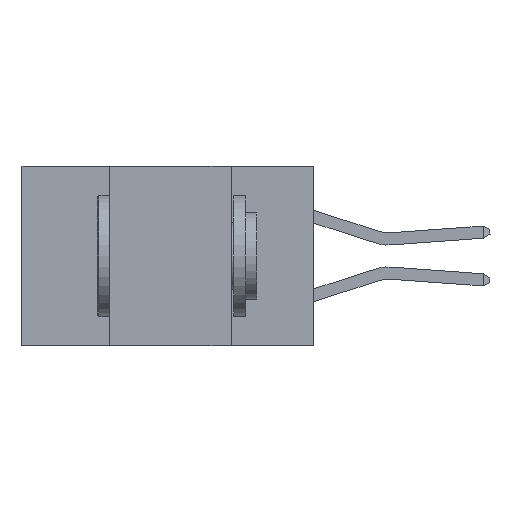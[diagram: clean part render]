
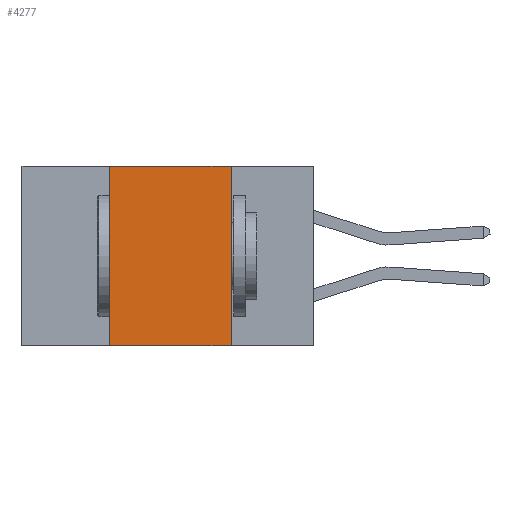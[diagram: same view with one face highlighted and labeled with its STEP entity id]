
A CAD part, left-side view. The second image highlights one B-rep face of the part: STEP entity #4277.
In plain terms, the highlighted planar face has unit normal (-1, 0, 0).
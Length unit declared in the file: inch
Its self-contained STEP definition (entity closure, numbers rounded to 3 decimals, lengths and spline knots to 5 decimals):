
#443 = EDGE_CURVE ( 'NONE', #3996, #13075, #4246, .T. ) ;
#648 = AXIS2_PLACEMENT_3D ( 'NONE', #6887, #17113, #2607 ) ;
#1270 = CARTESIAN_POINT ( 'NONE',  ( 0., 0.17, 0. ) ) ;
#2012 = CARTESIAN_POINT ( 'NONE',  ( 0., 0.6, 0. ) ) ;
#2023 = EDGE_LOOP ( 'NONE', ( #3875, #4181, #4690, #10925 ) ) ;
#2097 = EDGE_CURVE ( 'NONE', #2943, #5993, #6501, .T. ) ;
#2547 = PLANE ( 'NONE',  #648 ) ;
#2607 = DIRECTION ( 'NONE',  ( 0., 0., -1. ) ) ;
#2943 = VERTEX_POINT ( 'NONE', #13710 ) ;
#3200 = CARTESIAN_POINT ( 'NONE',  ( 0., 0.17, 0. ) ) ;
#3426 = DIRECTION ( 'NONE',  ( 0., -1., 0. ) ) ;
#3869 = DIRECTION ( 'NONE',  ( 0., 0., 1. ) ) ;
#3875 = ORIENTED_EDGE ( 'NONE', *, *, #443, .F. ) ;
#3996 = VERTEX_POINT ( 'NONE', #3200 ) ;
#4126 = VECTOR ( 'NONE', #3426, 39.37008 ) ;
#4181 = ORIENTED_EDGE ( 'NONE', *, *, #14505, .F. ) ;
#4246 = LINE ( 'NONE', #1270, #5162 ) ;
#4277 = ADVANCED_FACE ( 'NONE', ( #12314 ), #2547, .F. ) ;
#4450 = CARTESIAN_POINT ( 'NONE',  ( 0., 0.42, 0. ) ) ;
#4690 = ORIENTED_EDGE ( 'NONE', *, *, #2097, .F. ) ;
#5162 = VECTOR ( 'NONE', #14356, 39.37008 ) ;
#5337 = VECTOR ( 'NONE', #7429, 39.37008 ) ;
#5881 = CARTESIAN_POINT ( 'NONE',  ( 0., 0.17, -0.37 ) ) ;
#5993 = VERTEX_POINT ( 'NONE', #4450 ) ;
#6501 = LINE ( 'NONE', #15559, #14306 ) ;
#6887 = CARTESIAN_POINT ( 'NONE',  ( 0., 0.6, 0. ) ) ;
#7429 = DIRECTION ( 'NONE',  ( 0., -1., 0. ) ) ;
#8698 = CARTESIAN_POINT ( 'NONE',  ( 0., 0.6, -0.37 ) ) ;
#10925 = ORIENTED_EDGE ( 'NONE', *, *, #17658, .T. ) ;
#12314 = FACE_OUTER_BOUND ( 'NONE', #2023, .T. ) ;
#13075 = VERTEX_POINT ( 'NONE', #5881 ) ;
#13710 = CARTESIAN_POINT ( 'NONE',  ( 0., 0.42, -0.37 ) ) ;
#14306 = VECTOR ( 'NONE', #3869, 39.37008 ) ;
#14356 = DIRECTION ( 'NONE',  ( 0., 0., -1. ) ) ;
#14505 = EDGE_CURVE ( 'NONE', #5993, #3996, #18591, .T. ) ;
#15559 = CARTESIAN_POINT ( 'NONE',  ( 0., 0.42, 0. ) ) ;
#17034 = LINE ( 'NONE', #8698, #5337 ) ;
#17113 = DIRECTION ( 'NONE',  ( 1., 0., 0. ) ) ;
#17658 = EDGE_CURVE ( 'NONE', #2943, #13075, #17034, .T. ) ;
#18591 = LINE ( 'NONE', #2012, #4126 ) ;
